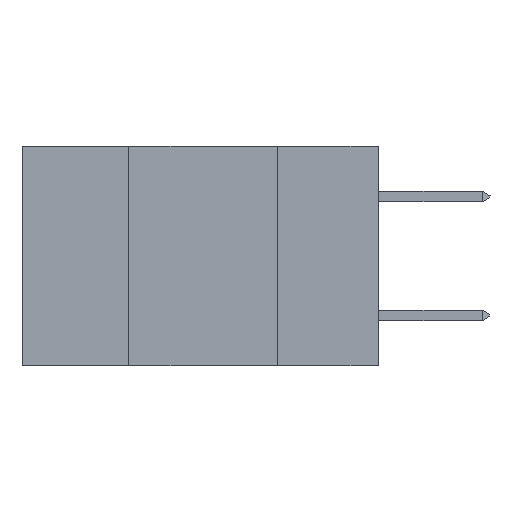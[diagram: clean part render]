
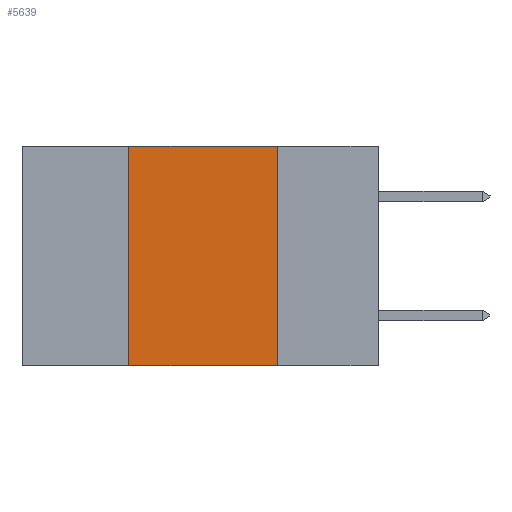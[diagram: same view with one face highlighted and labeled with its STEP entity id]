
A CAD part, left-side view. The second image highlights one B-rep face of the part: STEP entity #5639.
In plain terms, the highlighted planar face has unit normal (-1, 0, 0).
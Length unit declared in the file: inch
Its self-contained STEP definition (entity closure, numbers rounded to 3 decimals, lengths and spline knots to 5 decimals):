
#340 = PLANE ( 'NONE',  #5662 ) ;
#411 = EDGE_LOOP ( 'NONE', ( #3976, #3563, #1496, #1527 ) ) ;
#629 = DIRECTION ( 'NONE',  ( 0., -1., 0. ) ) ;
#1261 = CARTESIAN_POINT ( 'NONE',  ( 0., 0.6, 0. ) ) ;
#1447 = DIRECTION ( 'NONE',  ( 0., 0., 1. ) ) ;
#1496 = ORIENTED_EDGE ( 'NONE', *, *, #3249, .F. ) ;
#1527 = ORIENTED_EDGE ( 'NONE', *, *, #7084, .T. ) ;
#1825 = VECTOR ( 'NONE', #1447, 39.37008 ) ;
#2180 = VERTEX_POINT ( 'NONE', #2599 ) ;
#2376 = DIRECTION ( 'NONE',  ( 1., 0., 0. ) ) ;
#2436 = CARTESIAN_POINT ( 'NONE',  ( 0., 0.42, -0.37 ) ) ;
#2599 = CARTESIAN_POINT ( 'NONE',  ( 0., 0.17, -0.37 ) ) ;
#2676 = CARTESIAN_POINT ( 'NONE',  ( 0., 0.42, 0. ) ) ;
#2727 = CARTESIAN_POINT ( 'NONE',  ( 0., 0.6, -0.37 ) ) ;
#2951 = EDGE_CURVE ( 'NONE', #3183, #2180, #6943, .T. ) ;
#3013 = FACE_OUTER_BOUND ( 'NONE', #411, .T. ) ;
#3055 = CARTESIAN_POINT ( 'NONE',  ( 0., 0.6, 0. ) ) ;
#3183 = VERTEX_POINT ( 'NONE', #8449 ) ;
#3249 = EDGE_CURVE ( 'NONE', #6124, #7140, #3620, .T. ) ;
#3563 = ORIENTED_EDGE ( 'NONE', *, *, #4778, .F. ) ;
#3620 = LINE ( 'NONE', #7536, #1825 ) ;
#3679 = VECTOR ( 'NONE', #8347, 39.37008 ) ;
#3976 = ORIENTED_EDGE ( 'NONE', *, *, #2951, .F. ) ;
#4141 = DIRECTION ( 'NONE',  ( 0., -1., 0. ) ) ;
#4256 = VECTOR ( 'NONE', #4141, 39.37008 ) ;
#4377 = VECTOR ( 'NONE', #629, 39.37008 ) ;
#4756 = LINE ( 'NONE', #1261, #4377 ) ;
#4778 = EDGE_CURVE ( 'NONE', #7140, #3183, #4756, .T. ) ;
#5573 = DIRECTION ( 'NONE',  ( 0., 0., -1. ) ) ;
#5639 = ADVANCED_FACE ( 'NONE', ( #3013 ), #340, .F. ) ;
#5662 = AXIS2_PLACEMENT_3D ( 'NONE', #3055, #2376, #5573 ) ;
#6124 = VERTEX_POINT ( 'NONE', #2436 ) ;
#6858 = LINE ( 'NONE', #2727, #4256 ) ;
#6943 = LINE ( 'NONE', #8224, #3679 ) ;
#7084 = EDGE_CURVE ( 'NONE', #6124, #2180, #6858, .T. ) ;
#7140 = VERTEX_POINT ( 'NONE', #2676 ) ;
#7536 = CARTESIAN_POINT ( 'NONE',  ( 0., 0.42, -0.37 ) ) ;
#8224 = CARTESIAN_POINT ( 'NONE',  ( 0., 0.17, -0.37 ) ) ;
#8347 = DIRECTION ( 'NONE',  ( 0., 0., -1. ) ) ;
#8449 = CARTESIAN_POINT ( 'NONE',  ( 0., 0.17, 0. ) ) ;
